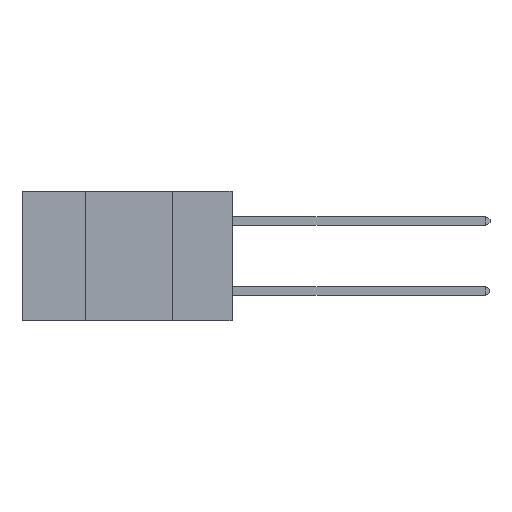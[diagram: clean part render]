
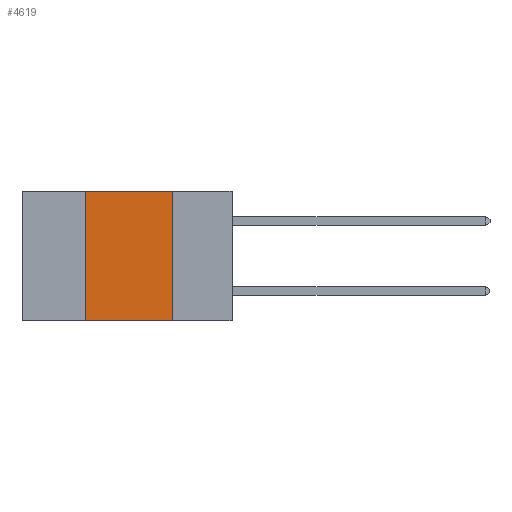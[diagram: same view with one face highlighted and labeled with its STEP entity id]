
A CAD part, left-side view. The second image highlights one B-rep face of the part: STEP entity #4619.
In plain terms, the highlighted planar face has unit normal (-1, 0, 0).
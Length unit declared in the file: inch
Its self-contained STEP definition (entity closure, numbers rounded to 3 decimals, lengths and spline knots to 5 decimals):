
#213 = EDGE_CURVE ( 'NONE', #10256, #1803, #2806, .T. ) ;
#484 = VERTEX_POINT ( 'NONE', #10812 ) ;
#574 = DIRECTION ( 'NONE',  ( 0., 0., -1. ) ) ;
#748 = DIRECTION ( 'NONE',  ( 1., 0., 0. ) ) ;
#1034 = PLANE ( 'NONE',  #3550 ) ;
#1127 = VERTEX_POINT ( 'NONE', #10277 ) ;
#1435 = CARTESIAN_POINT ( 'NONE',  ( 0., 0.6, 0. ) ) ;
#1737 = DIRECTION ( 'NONE',  ( 0., 0., 1. ) ) ;
#1803 = VERTEX_POINT ( 'NONE', #10569 ) ;
#2806 = LINE ( 'NONE', #8574, #9543 ) ;
#2930 = VECTOR ( 'NONE', #4178, 39.37008 ) ;
#3250 = DIRECTION ( 'NONE',  ( 0., 0., -1. ) ) ;
#3550 = AXIS2_PLACEMENT_3D ( 'NONE', #1435, #748, #574 ) ;
#3990 = LINE ( 'NONE', #5828, #10081 ) ;
#4178 = DIRECTION ( 'NONE',  ( 0., -1., 0. ) ) ;
#4379 = CARTESIAN_POINT ( 'NONE',  ( 0., 0.42, 0. ) ) ;
#4619 = ADVANCED_FACE ( 'NONE', ( #6144 ), #1034, .F. ) ;
#5077 = CARTESIAN_POINT ( 'NONE',  ( 0., 0.6, -0.37 ) ) ;
#5167 = EDGE_CURVE ( 'NONE', #1803, #1127, #3990, .T. ) ;
#5828 = CARTESIAN_POINT ( 'NONE',  ( 0., 0.17, 0. ) ) ;
#5866 = ORIENTED_EDGE ( 'NONE', *, *, #5167, .F. ) ;
#6135 = ORIENTED_EDGE ( 'NONE', *, *, #9034, .F. ) ;
#6144 = FACE_OUTER_BOUND ( 'NONE', #10332, .T. ) ;
#6551 = CARTESIAN_POINT ( 'NONE',  ( 0., 0.42, 0. ) ) ;
#7229 = LINE ( 'NONE', #4379, #9659 ) ;
#8337 = ORIENTED_EDGE ( 'NONE', *, *, #9579, .T. ) ;
#8574 = CARTESIAN_POINT ( 'NONE',  ( 0., 0.6, 0. ) ) ;
#9034 = EDGE_CURVE ( 'NONE', #484, #10256, #7229, .T. ) ;
#9543 = VECTOR ( 'NONE', #11023, 39.37008 ) ;
#9579 = EDGE_CURVE ( 'NONE', #484, #1127, #9649, .T. ) ;
#9649 = LINE ( 'NONE', #5077, #2930 ) ;
#9659 = VECTOR ( 'NONE', #1737, 39.37008 ) ;
#10081 = VECTOR ( 'NONE', #3250, 39.37008 ) ;
#10221 = ORIENTED_EDGE ( 'NONE', *, *, #213, .F. ) ;
#10256 = VERTEX_POINT ( 'NONE', #6551 ) ;
#10277 = CARTESIAN_POINT ( 'NONE',  ( 0., 0.17, -0.37 ) ) ;
#10332 = EDGE_LOOP ( 'NONE', ( #5866, #10221, #6135, #8337 ) ) ;
#10569 = CARTESIAN_POINT ( 'NONE',  ( 0., 0.17, 0. ) ) ;
#10812 = CARTESIAN_POINT ( 'NONE',  ( 0., 0.42, -0.37 ) ) ;
#11023 = DIRECTION ( 'NONE',  ( 0., -1., 0. ) ) ;
